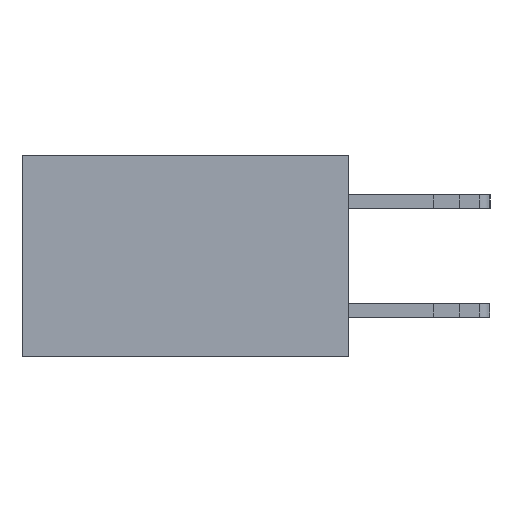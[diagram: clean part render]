
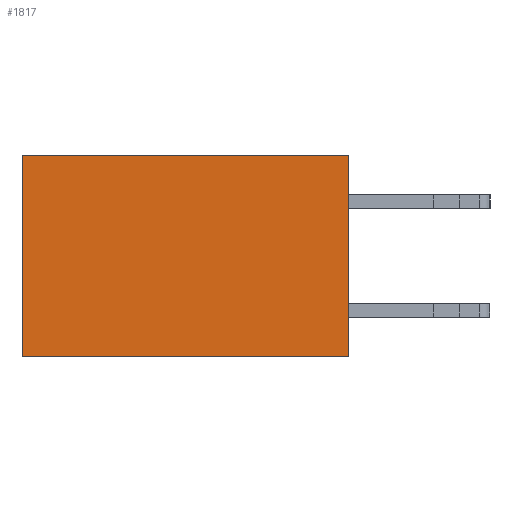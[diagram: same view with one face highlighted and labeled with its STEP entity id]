
A CAD part, left-side view. The second image highlights one B-rep face of the part: STEP entity #1817.
In plain terms, the highlighted planar face has unit normal (-1, 0, 0).
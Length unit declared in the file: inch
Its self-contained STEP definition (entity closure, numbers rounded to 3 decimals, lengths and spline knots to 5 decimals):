
#289 = CARTESIAN_POINT ( 'NONE',  ( 0.298, 0., 0. ) ) ;
#290 = CARTESIAN_POINT ( 'NONE',  ( 0.298, 0., 0. ) ) ;
#336 = ORIENTED_EDGE ( 'NONE', *, *, #16007, .F. ) ;
#1543 = DIRECTION ( 'NONE',  ( 0., 1., 0. ) ) ;
#1558 = CARTESIAN_POINT ( 'NONE',  ( 0.298, 0., 0. ) ) ;
#1578 = PLANE ( 'NONE',  #7226 ) ;
#1817 = ADVANCED_FACE ( 'NONE', ( #8165 ), #1578, .F. ) ;
#1983 = VECTOR ( 'NONE', #1543, 39.37008 ) ;
#2458 = CARTESIAN_POINT ( 'NONE',  ( 0.298, 0.6, 0. ) ) ;
#4283 = VECTOR ( 'NONE', #5358, 39.37008 ) ;
#4434 = ORIENTED_EDGE ( 'NONE', *, *, #5420, .F. ) ;
#5213 = CARTESIAN_POINT ( 'NONE',  ( 0.298, 0., -0.37 ) ) ;
#5358 = DIRECTION ( 'NONE',  ( 0., 1., 0. ) ) ;
#5420 = EDGE_CURVE ( 'NONE', #14358, #6986, #8011, .T. ) ;
#5532 = DIRECTION ( 'NONE',  ( 1., 0., 0. ) ) ;
#5670 = LINE ( 'NONE', #289, #1983 ) ;
#6493 = ORIENTED_EDGE ( 'NONE', *, *, #12824, .T. ) ;
#6767 = DIRECTION ( 'NONE',  ( 0., 0., -1. ) ) ;
#6986 = VERTEX_POINT ( 'NONE', #7192 ) ;
#7036 = VERTEX_POINT ( 'NONE', #13554 ) ;
#7192 = CARTESIAN_POINT ( 'NONE',  ( 0.298, 0.6, -0.37 ) ) ;
#7226 = AXIS2_PLACEMENT_3D ( 'NONE', #1558, #5532, #9535 ) ;
#8011 = LINE ( 'NONE', #5213, #4283 ) ;
#8165 = FACE_OUTER_BOUND ( 'NONE', #9810, .T. ) ;
#8973 = DIRECTION ( 'NONE',  ( 0., 0., -1. ) ) ;
#9062 = VERTEX_POINT ( 'NONE', #2458 ) ;
#9213 = CARTESIAN_POINT ( 'NONE',  ( 0.298, 0., -0.37 ) ) ;
#9535 = DIRECTION ( 'NONE',  ( 0., 0., -1. ) ) ;
#9608 = ORIENTED_EDGE ( 'NONE', *, *, #12013, .T. ) ;
#9810 = EDGE_LOOP ( 'NONE', ( #9608, #4434, #336, #6493 ) ) ;
#10807 = VECTOR ( 'NONE', #6767, 39.37008 ) ;
#12013 = EDGE_CURVE ( 'NONE', #9062, #6986, #13750, .T. ) ;
#12143 = VECTOR ( 'NONE', #8973, 39.37008 ) ;
#12524 = LINE ( 'NONE', #290, #12143 ) ;
#12824 = EDGE_CURVE ( 'NONE', #7036, #9062, #5670, .T. ) ;
#13554 = CARTESIAN_POINT ( 'NONE',  ( 0.298, 0., 0. ) ) ;
#13750 = LINE ( 'NONE', #14285, #10807 ) ;
#14285 = CARTESIAN_POINT ( 'NONE',  ( 0.298, 0.6, 0. ) ) ;
#14358 = VERTEX_POINT ( 'NONE', #9213 ) ;
#16007 = EDGE_CURVE ( 'NONE', #7036, #14358, #12524, .T. ) ;
